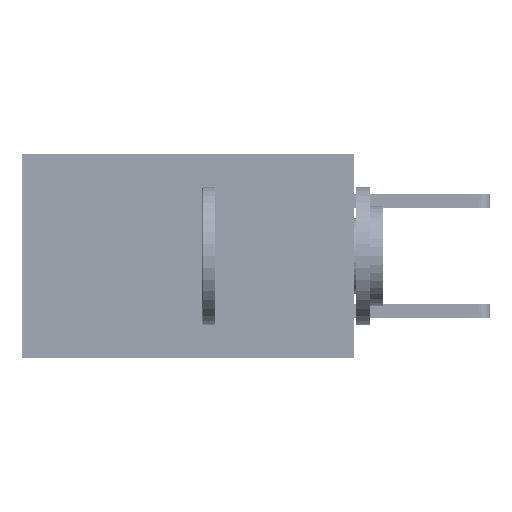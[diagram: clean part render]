
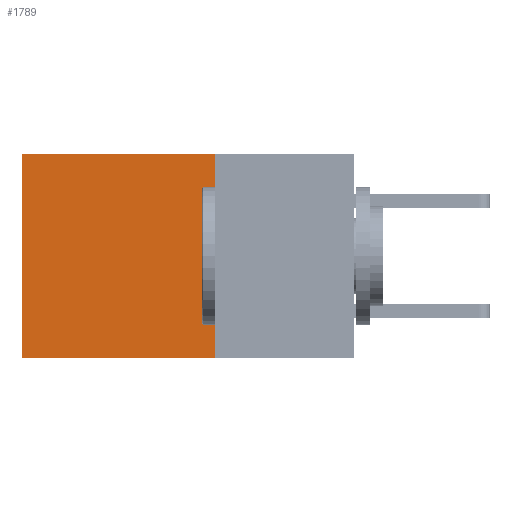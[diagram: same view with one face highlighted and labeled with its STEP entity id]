
A CAD part, left-side view. The second image highlights one B-rep face of the part: STEP entity #1789.
In plain terms, the highlighted planar face has unit normal (-1, 0, 0).
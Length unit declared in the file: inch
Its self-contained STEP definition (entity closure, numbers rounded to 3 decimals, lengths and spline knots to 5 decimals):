
#1686 = FACE_OUTER_BOUND ( 'NONE', #28314, .T. ) ;
#1789 = ADVANCED_FACE ( 'NONE', ( #1686 ), #28230, .F. ) ;
#4113 = CARTESIAN_POINT ( 'NONE',  ( 0.2875, 0.6, 0. ) ) ;
#4453 = DIRECTION ( 'NONE',  ( 0., 0., -1. ) ) ;
#7130 = VERTEX_POINT ( 'NONE', #50864 ) ;
#8260 = ORIENTED_EDGE ( 'NONE', *, *, #41268, .F. ) ;
#9730 = VECTOR ( 'NONE', #11642, 39.37008 ) ;
#10478 = CARTESIAN_POINT ( 'NONE',  ( 0.2875, 0.25, -0.37 ) ) ;
#11010 = LINE ( 'NONE', #40631, #9730 ) ;
#11152 = VECTOR ( 'NONE', #25013, 39.37008 ) ;
#11642 = DIRECTION ( 'NONE',  ( 0., 1., 0. ) ) ;
#14704 = EDGE_CURVE ( 'NONE', #37727, #25399, #43376, .T. ) ;
#15936 = EDGE_CURVE ( 'NONE', #7130, #37727, #11010, .T. ) ;
#16719 = DIRECTION ( 'NONE',  ( 1., 0., 0. ) ) ;
#21014 = LINE ( 'NONE', #10478, #48883 ) ;
#21322 = CARTESIAN_POINT ( 'NONE',  ( 0.2875, 0.25, -0.37 ) ) ;
#24478 = CARTESIAN_POINT ( 'NONE',  ( 0.2875, 0.25, 0. ) ) ;
#24923 = EDGE_CURVE ( 'NONE', #7130, #41593, #37191, .T. ) ;
#25013 = DIRECTION ( 'NONE',  ( 0., 0., -1. ) ) ;
#25399 = VERTEX_POINT ( 'NONE', #36786 ) ;
#26232 = DIRECTION ( 'NONE',  ( 0., 0., -1. ) ) ;
#27098 = DIRECTION ( 'NONE',  ( 0., 1., 0. ) ) ;
#27557 = CARTESIAN_POINT ( 'NONE',  ( 0.2875, 0.6, 0. ) ) ;
#28230 = PLANE ( 'NONE',  #40195 ) ;
#28314 = EDGE_LOOP ( 'NONE', ( #50280, #8260, #35424, #38886 ) ) ;
#35424 = ORIENTED_EDGE ( 'NONE', *, *, #24923, .F. ) ;
#36786 = CARTESIAN_POINT ( 'NONE',  ( 0.2875, 0.6, -0.37 ) ) ;
#37191 = LINE ( 'NONE', #42823, #38481 ) ;
#37727 = VERTEX_POINT ( 'NONE', #27557 ) ;
#38481 = VECTOR ( 'NONE', #26232, 39.37008 ) ;
#38886 = ORIENTED_EDGE ( 'NONE', *, *, #15936, .T. ) ;
#40195 = AXIS2_PLACEMENT_3D ( 'NONE', #24478, #16719, #4453 ) ;
#40631 = CARTESIAN_POINT ( 'NONE',  ( 0.2875, 0.25, 0. ) ) ;
#41268 = EDGE_CURVE ( 'NONE', #41593, #25399, #21014, .T. ) ;
#41593 = VERTEX_POINT ( 'NONE', #21322 ) ;
#42823 = CARTESIAN_POINT ( 'NONE',  ( 0.2875, 0.25, 0. ) ) ;
#43376 = LINE ( 'NONE', #4113, #11152 ) ;
#48883 = VECTOR ( 'NONE', #27098, 39.37008 ) ;
#50280 = ORIENTED_EDGE ( 'NONE', *, *, #14704, .T. ) ;
#50864 = CARTESIAN_POINT ( 'NONE',  ( 0.2875, 0.25, 0. ) ) ;
